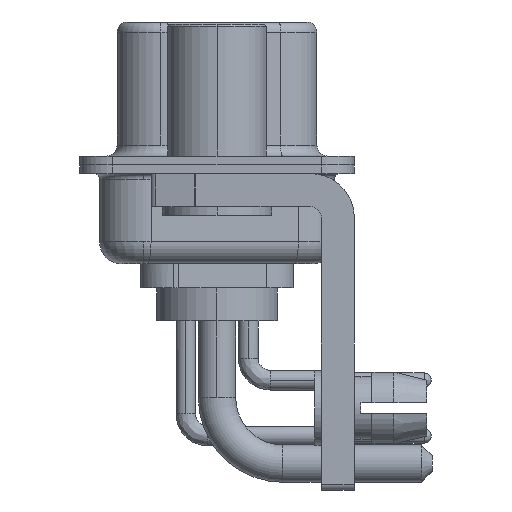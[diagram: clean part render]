
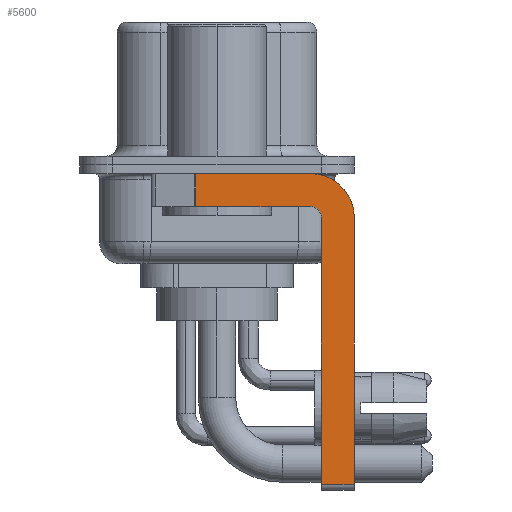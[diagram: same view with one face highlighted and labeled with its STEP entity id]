
A CAD part, left-side view. The second image highlights one B-rep face of the part: STEP entity #5600.
In plain terms, the highlighted planar face has unit normal (-1, 0, 0).
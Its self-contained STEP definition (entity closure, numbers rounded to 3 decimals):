
#43 = VERTEX_POINT ( 'NONE', #1998 ) ;
#959 = EDGE_CURVE ( 'NONE', #13428, #4263, #10378, .T. ) ;
#1076 = CARTESIAN_POINT ( 'NONE',  ( -2.9, -6.25, -2.4 ) ) ;
#1243 = DIRECTION ( 'NONE',  ( 0., 0., -1. ) ) ;
#1583 = LINE ( 'NONE', #11296, #9827 ) ;
#1604 = VECTOR ( 'NONE', #28774, 1000. ) ;
#1744 = CARTESIAN_POINT ( 'NONE',  ( -2.9, -4.25, -1.9 ) ) ;
#1998 = CARTESIAN_POINT ( 'NONE',  ( -2.9, 0.978, -1.9 ) ) ;
#2681 = LINE ( 'NONE', #21309, #22420 ) ;
#2788 = VERTEX_POINT ( 'NONE', #18599 ) ;
#3341 = LINE ( 'NONE', #3645, #25710 ) ;
#3645 = CARTESIAN_POINT ( 'NONE',  ( -2.9, 3., -0.4 ) ) ;
#3793 = ORIENTED_EDGE ( 'NONE', *, *, #8779, .F. ) ;
#4263 = VERTEX_POINT ( 'NONE', #1076 ) ;
#4292 = DIRECTION ( 'NONE',  ( 0., 0., -1. ) ) ;
#4429 = DIRECTION ( 'NONE',  ( -1., 0., 0. ) ) ;
#4978 = CARTESIAN_POINT ( 'NONE',  ( -2.9, -4.25, -14.55 ) ) ;
#5600 = ADVANCED_FACE ( 'NONE', ( #11098 ), #28582, .F. ) ;
#6173 = ORIENTED_EDGE ( 'NONE', *, *, #959, .F. ) ;
#6184 = DIRECTION ( 'NONE',  ( 0., -1., 0. ) ) ;
#7396 = EDGE_CURVE ( 'NONE', #19118, #27709, #21358, .T. ) ;
#7444 = VECTOR ( 'NONE', #27513, 1000. ) ;
#8461 = VERTEX_POINT ( 'NONE', #24974 ) ;
#8779 = EDGE_CURVE ( 'NONE', #27709, #43, #23982, .T. ) ;
#9827 = VECTOR ( 'NONE', #4292, 1000. ) ;
#9993 = EDGE_CURVE ( 'NONE', #26384, #19118, #2681, .T. ) ;
#10139 = AXIS2_PLACEMENT_3D ( 'NONE', #25563, #18881, #28109 ) ;
#10378 = CIRCLE ( 'NONE', #22025, 2. ) ;
#11098 = FACE_OUTER_BOUND ( 'NONE', #30672, .T. ) ;
#11296 = CARTESIAN_POINT ( 'NONE',  ( -2.9, -6.25, -2.4 ) ) ;
#11317 = CARTESIAN_POINT ( 'NONE',  ( -2.9, -4.25, -2.4 ) ) ;
#11746 = CARTESIAN_POINT ( 'NONE',  ( -2.9, -4.25, -1.9 ) ) ;
#11913 = EDGE_CURVE ( 'NONE', #4263, #2788, #1583, .T. ) ;
#13338 = CARTESIAN_POINT ( 'NONE',  ( -2.9, 0.978, -1.9 ) ) ;
#13428 = VERTEX_POINT ( 'NONE', #14649 ) ;
#13481 = EDGE_CURVE ( 'NONE', #8461, #43, #25112, .T. ) ;
#13886 = ORIENTED_EDGE ( 'NONE', *, *, #11913, .F. ) ;
#14649 = CARTESIAN_POINT ( 'NONE',  ( -2.9, -4.25, -0.4 ) ) ;
#15228 = ORIENTED_EDGE ( 'NONE', *, *, #7396, .F. ) ;
#16345 = CARTESIAN_POINT ( 'NONE',  ( -2.9, -4.25, -2.4 ) ) ;
#18572 = ORIENTED_EDGE ( 'NONE', *, *, #23066, .F. ) ;
#18599 = CARTESIAN_POINT ( 'NONE',  ( -2.9, -6.25, -14.55 ) ) ;
#18635 = DIRECTION ( 'NONE',  ( 0., 0., -1. ) ) ;
#18793 = DIRECTION ( 'NONE',  ( 1., 0., 0. ) ) ;
#18881 = DIRECTION ( 'NONE',  ( 1., 0., 0. ) ) ;
#19118 = VERTEX_POINT ( 'NONE', #28048 ) ;
#19568 = VECTOR ( 'NONE', #1243, 1000. ) ;
#21309 = CARTESIAN_POINT ( 'NONE',  ( -2.9, -4.75, -14.8 ) ) ;
#21358 = CIRCLE ( 'NONE', #21863, 0.5 ) ;
#21863 = AXIS2_PLACEMENT_3D ( 'NONE', #16345, #4429, #23499 ) ;
#21991 = ORIENTED_EDGE ( 'NONE', *, *, #9993, .F. ) ;
#21998 = LINE ( 'NONE', #4978, #7444 ) ;
#22025 = AXIS2_PLACEMENT_3D ( 'NONE', #11317, #18793, #18635 ) ;
#22420 = VECTOR ( 'NONE', #31017, 1000. ) ;
#23007 = ORIENTED_EDGE ( 'NONE', *, *, #28427, .T. ) ;
#23066 = EDGE_CURVE ( 'NONE', #8461, #13428, #3341, .T. ) ;
#23499 = DIRECTION ( 'NONE',  ( 0., 0., 1. ) ) ;
#23982 = LINE ( 'NONE', #11746, #1604 ) ;
#24974 = CARTESIAN_POINT ( 'NONE',  ( -2.9, 0.978, -0.4 ) ) ;
#25112 = LINE ( 'NONE', #13338, #19568 ) ;
#25563 = CARTESIAN_POINT ( 'NONE',  ( -2.9, -4.25, -2.4 ) ) ;
#25710 = VECTOR ( 'NONE', #6184, 1000. ) ;
#26078 = CARTESIAN_POINT ( 'NONE',  ( -2.9, -4.75, -14.55 ) ) ;
#26384 = VERTEX_POINT ( 'NONE', #26078 ) ;
#27513 = DIRECTION ( 'NONE',  ( 0., -1., 0. ) ) ;
#27709 = VERTEX_POINT ( 'NONE', #1744 ) ;
#28048 = CARTESIAN_POINT ( 'NONE',  ( -2.9, -4.75, -2.4 ) ) ;
#28109 = DIRECTION ( 'NONE',  ( 0., 0., -1. ) ) ;
#28427 = EDGE_CURVE ( 'NONE', #26384, #2788, #21998, .T. ) ;
#28582 = PLANE ( 'NONE',  #10139 ) ;
#28774 = DIRECTION ( 'NONE',  ( 0., 1., 0. ) ) ;
#29958 = ORIENTED_EDGE ( 'NONE', *, *, #13481, .T. ) ;
#30672 = EDGE_LOOP ( 'NONE', ( #18572, #29958, #3793, #15228, #21991, #23007, #13886, #6173 ) ) ;
#31017 = DIRECTION ( 'NONE',  ( 0., 0., 1. ) ) ;
